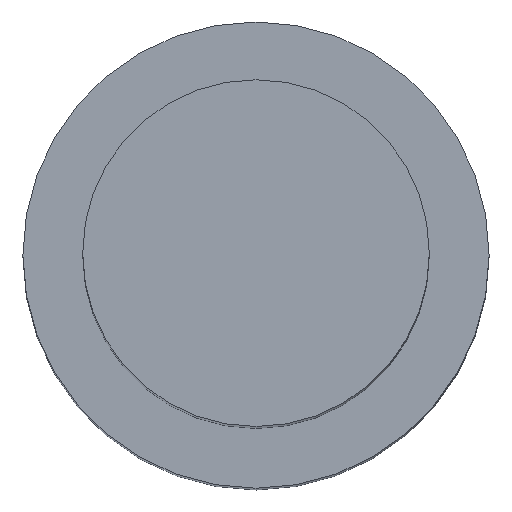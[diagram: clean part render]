
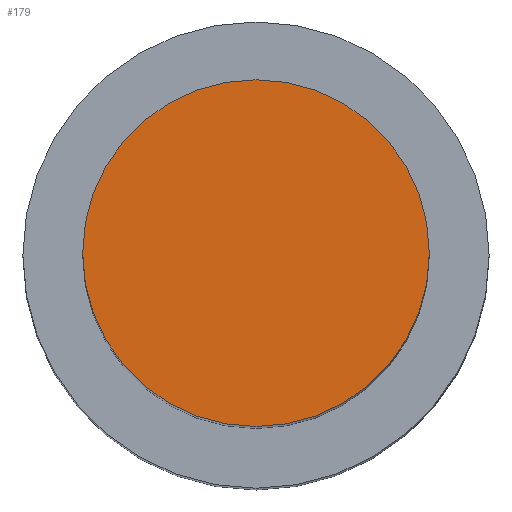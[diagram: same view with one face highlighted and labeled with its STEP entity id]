
A CAD part, top view. The second image highlights one B-rep face of the part: STEP entity #179.
In plain terms, the highlighted planar face has unit normal (0, 0, 1).
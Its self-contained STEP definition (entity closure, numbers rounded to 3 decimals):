
#56 = ORIENTED_EDGE ( 'NONE', *, *, #129, .T. ) ;
#82 = VERTEX_POINT ( 'NONE', #163 ) ;
#84 = FACE_OUTER_BOUND ( 'NONE', #236, .T. ) ;
#94 = DIRECTION ( 'NONE',  ( 0., 0., 1. ) ) ;
#129 = EDGE_CURVE ( 'NONE', #82, #82, #285, .T. ) ;
#137 = DIRECTION ( 'NONE',  ( 0., 0., 1. ) ) ;
#163 = CARTESIAN_POINT ( 'NONE',  ( -22.115, -13.375, 18.433 ) ) ;
#165 = CARTESIAN_POINT ( 'NONE',  ( -25.015, -13.375, 18.433 ) ) ;
#179 = ADVANCED_FACE ( 'NONE', ( #84 ), #290, .T. ) ;
#206 = AXIS2_PLACEMENT_3D ( 'NONE', #214, #94, #266 ) ;
#214 = CARTESIAN_POINT ( 'NONE',  ( -25.015, -13.375, 18.433 ) ) ;
#236 = EDGE_LOOP ( 'NONE', ( #56 ) ) ;
#251 = AXIS2_PLACEMENT_3D ( 'NONE', #165, #137, #263 ) ;
#263 = DIRECTION ( 'NONE',  ( 1., 0., 0. ) ) ;
#266 = DIRECTION ( 'NONE',  ( 1., 0., 0. ) ) ;
#285 = CIRCLE ( 'NONE', #251, 2.9 ) ;
#290 = PLANE ( 'NONE',  #206 ) ;
